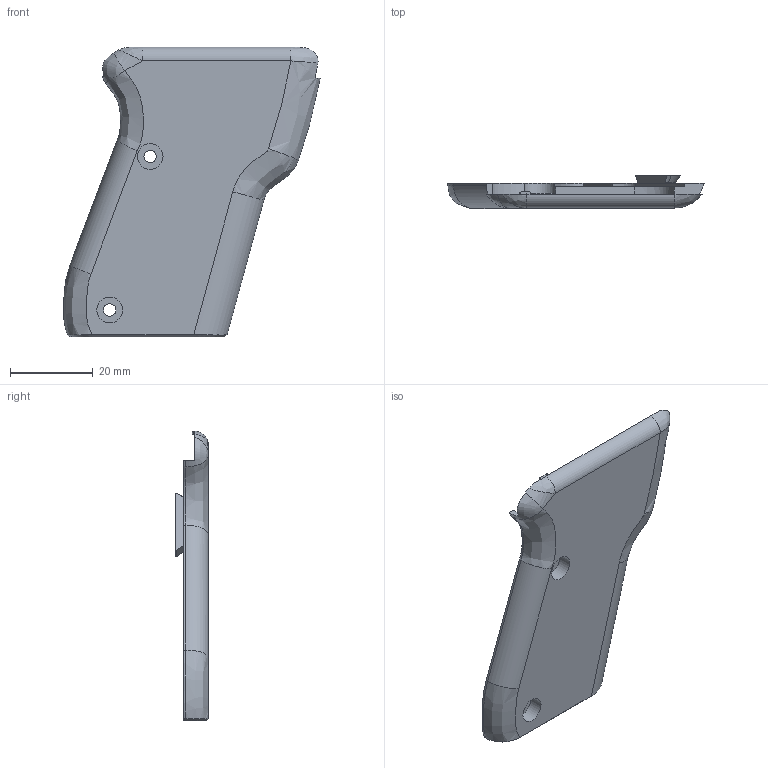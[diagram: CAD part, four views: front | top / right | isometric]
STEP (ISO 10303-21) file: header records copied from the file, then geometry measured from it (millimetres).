
FILE_DESCRIPTION(/* description */ (''),/* implementation_level */ '2;1');
FILE_NAME(/* name */ 'right_grip_finalj.step',/* time_stamp */ '2021-09-19T17:09:42-04:00',/* author */ (''),/* organization */ (''),/* preprocessor_version */ 'ST-DEVELOPER v18.1',/* originating_system */ 'Autodesk Translation Framework v10.10.0.1391',/* authorisation */ '');
FILE_SCHEMA (('AUTOMOTIVE_DESIGN { 1 0 10303 214 3 1 1 }'));
Length unit declared in the file: millimetre
Products named in the file (1): right_grip
Bounding box: 61.89 x 7.9 x 69.91 mm (x, y, z)
Volume: 13614.3 mm3; surface area: 7763.6 mm2
Topology: 1 solids, 1 shells, 73 faces, 191 edges, 121 vertices
Faces by surface type: plane 32, bspline 24, cylinder 15, torus 2
Full cylindrical faces by diameter (mm): 3 x2, 6.2 x2
Entity records: 3686 total; most frequent: CARTESIAN_POINT 2029, ORIENTED_EDGE 380, DIRECTION 267, EDGE_CURVE 190, VERTEX_POINT 121, LINE 97, VECTOR 97, AXIS2_PLACEMENT_3D 85
